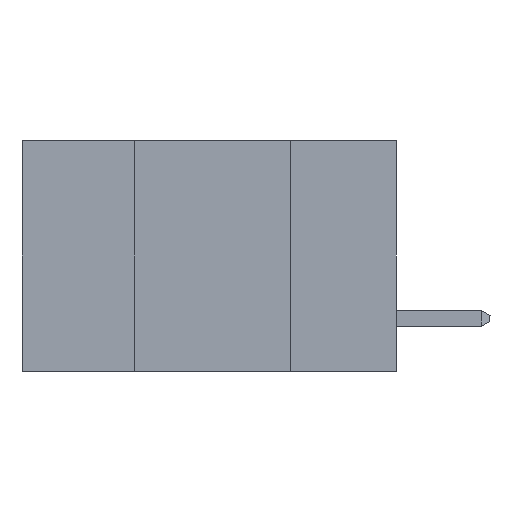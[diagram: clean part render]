
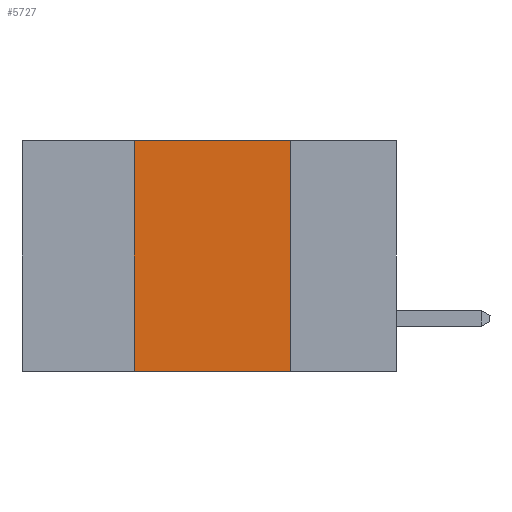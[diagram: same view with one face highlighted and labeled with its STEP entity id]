
A CAD part, left-side view. The second image highlights one B-rep face of the part: STEP entity #5727.
In plain terms, the highlighted planar face has unit normal (-1, 0, 0).
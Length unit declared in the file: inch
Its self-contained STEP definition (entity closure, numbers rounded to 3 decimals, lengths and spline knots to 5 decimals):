
#176 = CARTESIAN_POINT ( 'NONE',  ( 0., 0.6, -0.37 ) ) ;
#524 = FACE_OUTER_BOUND ( 'NONE', #7732, .T. ) ;
#1560 = VERTEX_POINT ( 'NONE', #8629 ) ;
#1575 = VERTEX_POINT ( 'NONE', #6485 ) ;
#1580 = EDGE_CURVE ( 'NONE', #2672, #1575, #6973, .T. ) ;
#2094 = LINE ( 'NONE', #9687, #7295 ) ;
#2554 = ORIENTED_EDGE ( 'NONE', *, *, #4048, .F. ) ;
#2632 = EDGE_CURVE ( 'NONE', #6186, #1560, #6417, .T. ) ;
#2672 = VERTEX_POINT ( 'NONE', #11913 ) ;
#3209 = DIRECTION ( 'NONE',  ( 0., -1., 0. ) ) ;
#3282 = DIRECTION ( 'NONE',  ( 0., -1., 0. ) ) ;
#3469 = VECTOR ( 'NONE', #3209, 39.37008 ) ;
#4048 = EDGE_CURVE ( 'NONE', #1560, #2672, #2094, .T. ) ;
#4162 = DIRECTION ( 'NONE',  ( 0., 0., 1. ) ) ;
#5727 = ADVANCED_FACE ( 'NONE', ( #524 ), #13570, .F. ) ;
#6181 = ORIENTED_EDGE ( 'NONE', *, *, #7184, .T. ) ;
#6186 = VERTEX_POINT ( 'NONE', #7011 ) ;
#6417 = LINE ( 'NONE', #8419, #7748 ) ;
#6485 = CARTESIAN_POINT ( 'NONE',  ( 0., 0.17, -0.37 ) ) ;
#6973 = LINE ( 'NONE', #8064, #9524 ) ;
#7011 = CARTESIAN_POINT ( 'NONE',  ( 0., 0.42, -0.37 ) ) ;
#7184 = EDGE_CURVE ( 'NONE', #6186, #1575, #9968, .T. ) ;
#7295 = VECTOR ( 'NONE', #3282, 39.37008 ) ;
#7732 = EDGE_LOOP ( 'NONE', ( #9220, #2554, #9548, #6181 ) ) ;
#7748 = VECTOR ( 'NONE', #4162, 39.37008 ) ;
#8064 = CARTESIAN_POINT ( 'NONE',  ( 0., 0.17, -0.37 ) ) ;
#8115 = DIRECTION ( 'NONE',  ( 0., 0., -1. ) ) ;
#8419 = CARTESIAN_POINT ( 'NONE',  ( 0., 0.42, -0.37 ) ) ;
#8629 = CARTESIAN_POINT ( 'NONE',  ( 0., 0.42, 0. ) ) ;
#9051 = DIRECTION ( 'NONE',  ( 0., 0., -1. ) ) ;
#9181 = CARTESIAN_POINT ( 'NONE',  ( 0., 0.6, 0. ) ) ;
#9220 = ORIENTED_EDGE ( 'NONE', *, *, #1580, .F. ) ;
#9524 = VECTOR ( 'NONE', #9051, 39.37008 ) ;
#9548 = ORIENTED_EDGE ( 'NONE', *, *, #2632, .F. ) ;
#9687 = CARTESIAN_POINT ( 'NONE',  ( 0., 0.6, 0. ) ) ;
#9774 = AXIS2_PLACEMENT_3D ( 'NONE', #9181, #13498, #8115 ) ;
#9968 = LINE ( 'NONE', #176, #3469 ) ;
#11913 = CARTESIAN_POINT ( 'NONE',  ( 0., 0.17, 0. ) ) ;
#13498 = DIRECTION ( 'NONE',  ( 1., 0., 0. ) ) ;
#13570 = PLANE ( 'NONE',  #9774 ) ;
